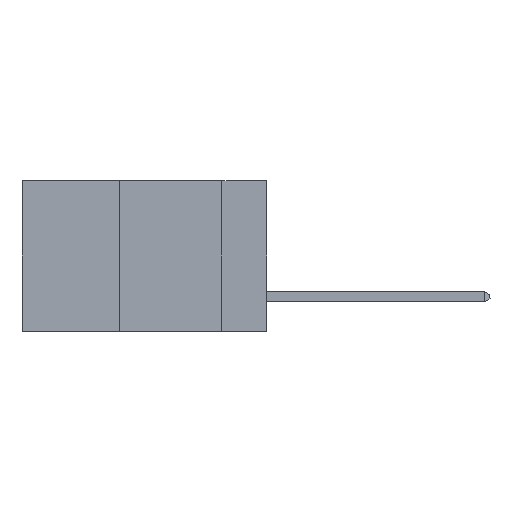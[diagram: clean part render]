
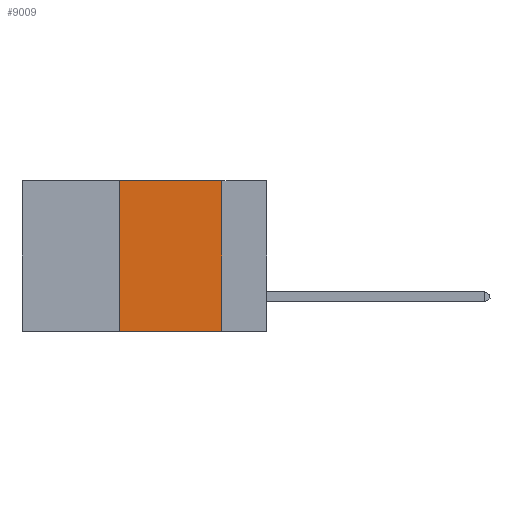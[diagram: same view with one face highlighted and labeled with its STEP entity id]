
A CAD part, left-side view. The second image highlights one B-rep face of the part: STEP entity #9009.
In plain terms, the highlighted planar face has unit normal (-1, 0, 0).
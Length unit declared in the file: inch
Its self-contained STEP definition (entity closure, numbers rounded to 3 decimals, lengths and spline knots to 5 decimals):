
#55 = CARTESIAN_POINT ( 'NONE',  ( 0., 0.6, -0.37 ) ) ;
#110 = LINE ( 'NONE', #6182, #4945 ) ;
#422 = VERTEX_POINT ( 'NONE', #10149 ) ;
#735 = DIRECTION ( 'NONE',  ( 1., 0., 0. ) ) ;
#811 = DIRECTION ( 'NONE',  ( 0., 0., 1. ) ) ;
#1227 = DIRECTION ( 'NONE',  ( 0., -1., 0. ) ) ;
#1335 = LINE ( 'NONE', #3146, #3813 ) ;
#1534 = CARTESIAN_POINT ( 'NONE',  ( 0., 0.36, 0. ) ) ;
#2135 = VERTEX_POINT ( 'NONE', #2378 ) ;
#2240 = ORIENTED_EDGE ( 'NONE', *, *, #5785, .F. ) ;
#2378 = CARTESIAN_POINT ( 'NONE',  ( 0., 0.36, 0. ) ) ;
#3129 = CARTESIAN_POINT ( 'NONE',  ( 0., 0.36, -0.37 ) ) ;
#3146 = CARTESIAN_POINT ( 'NONE',  ( 0., 0.6, 0. ) ) ;
#3328 = LINE ( 'NONE', #55, #5776 ) ;
#3632 = EDGE_CURVE ( 'NONE', #4105, #2135, #7089, .T. ) ;
#3633 = ORIENTED_EDGE ( 'NONE', *, *, #10436, .F. ) ;
#3813 = VECTOR ( 'NONE', #1227, 39.37008 ) ;
#3844 = CARTESIAN_POINT ( 'NONE',  ( 0., 0.11, -0.37 ) ) ;
#4105 = VERTEX_POINT ( 'NONE', #3129 ) ;
#4696 = VECTOR ( 'NONE', #811, 39.37008 ) ;
#4945 = VECTOR ( 'NONE', #10966, 39.37008 ) ;
#5460 = PLANE ( 'NONE',  #8208 ) ;
#5776 = VECTOR ( 'NONE', #7520, 39.37008 ) ;
#5785 = EDGE_CURVE ( 'NONE', #2135, #422, #1335, .T. ) ;
#6182 = CARTESIAN_POINT ( 'NONE',  ( 0., 0.11, 0. ) ) ;
#6189 = VERTEX_POINT ( 'NONE', #3844 ) ;
#6367 = CARTESIAN_POINT ( 'NONE',  ( 0., 0.6, 0. ) ) ;
#6970 = ORIENTED_EDGE ( 'NONE', *, *, #8610, .T. ) ;
#7042 = ORIENTED_EDGE ( 'NONE', *, *, #3632, .F. ) ;
#7089 = LINE ( 'NONE', #1534, #4696 ) ;
#7224 = DIRECTION ( 'NONE',  ( 0., 0., -1. ) ) ;
#7520 = DIRECTION ( 'NONE',  ( 0., -1., 0. ) ) ;
#8026 = EDGE_LOOP ( 'NONE', ( #3633, #2240, #7042, #6970 ) ) ;
#8208 = AXIS2_PLACEMENT_3D ( 'NONE', #6367, #735, #7224 ) ;
#8610 = EDGE_CURVE ( 'NONE', #4105, #6189, #3328, .T. ) ;
#9009 = ADVANCED_FACE ( 'NONE', ( #9886 ), #5460, .F. ) ;
#9886 = FACE_OUTER_BOUND ( 'NONE', #8026, .T. ) ;
#10149 = CARTESIAN_POINT ( 'NONE',  ( 0., 0.11, 0. ) ) ;
#10436 = EDGE_CURVE ( 'NONE', #422, #6189, #110, .T. ) ;
#10966 = DIRECTION ( 'NONE',  ( 0., 0., -1. ) ) ;
